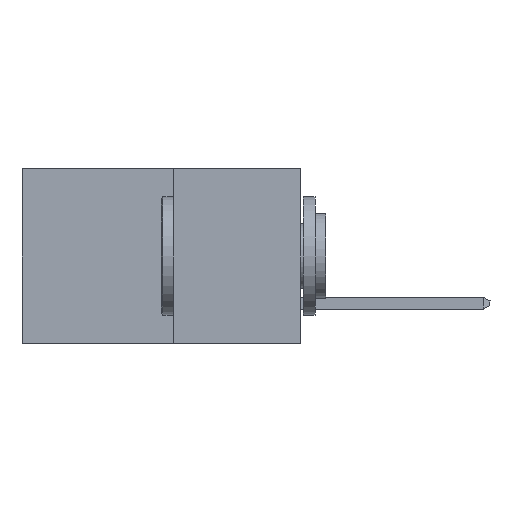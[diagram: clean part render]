
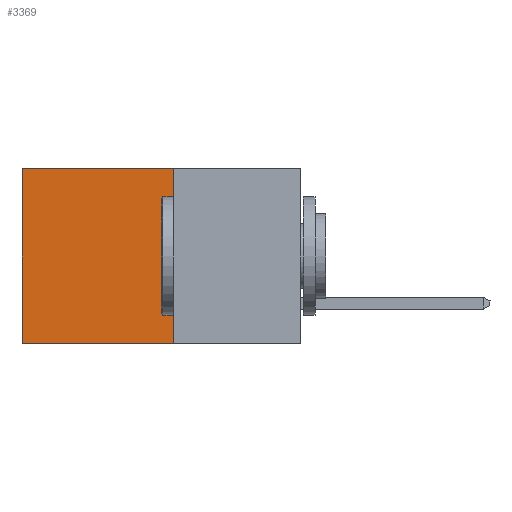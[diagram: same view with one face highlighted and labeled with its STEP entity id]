
A CAD part, left-side view. The second image highlights one B-rep face of the part: STEP entity #3369.
In plain terms, the highlighted planar face has unit normal (-1, 0, 0).
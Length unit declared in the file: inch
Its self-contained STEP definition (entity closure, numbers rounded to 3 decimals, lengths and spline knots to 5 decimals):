
#346 = VECTOR ( 'NONE', #9532, 39.37008 ) ;
#1127 = LINE ( 'NONE', #11704, #3586 ) ;
#1340 = VERTEX_POINT ( 'NONE', #4122 ) ;
#1895 = VERTEX_POINT ( 'NONE', #11166 ) ;
#2033 = ORIENTED_EDGE ( 'NONE', *, *, #8017, .T. ) ;
#2488 = EDGE_CURVE ( 'NONE', #5098, #1340, #13075, .T. ) ;
#2871 = CARTESIAN_POINT ( 'NONE',  ( 0.277, 0.27, -0.37 ) ) ;
#3369 = ADVANCED_FACE ( 'NONE', ( #10171 ), #11285, .F. ) ;
#3586 = VECTOR ( 'NONE', #9541, 39.37008 ) ;
#3850 = ORIENTED_EDGE ( 'NONE', *, *, #8998, .F. ) ;
#3867 = ORIENTED_EDGE ( 'NONE', *, *, #7310, .F. ) ;
#4122 = CARTESIAN_POINT ( 'NONE',  ( 0.277, 0.59, -0.37 ) ) ;
#4153 = EDGE_LOOP ( 'NONE', ( #10126, #3867, #3850, #2033 ) ) ;
#4335 = VECTOR ( 'NONE', #13903, 39.37008 ) ;
#5098 = VERTEX_POINT ( 'NONE', #14252 ) ;
#6669 = LINE ( 'NONE', #8452, #346 ) ;
#6967 = CARTESIAN_POINT ( 'NONE',  ( 0.277, 0.27, -0.37 ) ) ;
#7310 = EDGE_CURVE ( 'NONE', #8652, #1340, #7337, .T. ) ;
#7337 = LINE ( 'NONE', #2871, #4335 ) ;
#8017 = EDGE_CURVE ( 'NONE', #1895, #5098, #1127, .T. ) ;
#8452 = CARTESIAN_POINT ( 'NONE',  ( 0.277, 0.27, -0.37 ) ) ;
#8652 = VERTEX_POINT ( 'NONE', #6967 ) ;
#8998 = EDGE_CURVE ( 'NONE', #1895, #8652, #6669, .T. ) ;
#9532 = DIRECTION ( 'NONE',  ( 0., 0., -1. ) ) ;
#9541 = DIRECTION ( 'NONE',  ( 0., 1., 0. ) ) ;
#9862 = VECTOR ( 'NONE', #11952, 39.37008 ) ;
#9932 = AXIS2_PLACEMENT_3D ( 'NONE', #12037, #10806, #10727 ) ;
#10126 = ORIENTED_EDGE ( 'NONE', *, *, #2488, .T. ) ;
#10171 = FACE_OUTER_BOUND ( 'NONE', #4153, .T. ) ;
#10727 = DIRECTION ( 'NONE',  ( 0., 0., -1. ) ) ;
#10806 = DIRECTION ( 'NONE',  ( 1., 0., 0. ) ) ;
#11166 = CARTESIAN_POINT ( 'NONE',  ( 0.277, 0.27, 0. ) ) ;
#11285 = PLANE ( 'NONE',  #9932 ) ;
#11704 = CARTESIAN_POINT ( 'NONE',  ( 0.277, 0.27, 0. ) ) ;
#11767 = CARTESIAN_POINT ( 'NONE',  ( 0.277, 0.59, -0.37 ) ) ;
#11952 = DIRECTION ( 'NONE',  ( 0., 0., -1. ) ) ;
#12037 = CARTESIAN_POINT ( 'NONE',  ( 0.277, 0.27, -0.37 ) ) ;
#13075 = LINE ( 'NONE', #11767, #9862 ) ;
#13903 = DIRECTION ( 'NONE',  ( 0., 1., 0. ) ) ;
#14252 = CARTESIAN_POINT ( 'NONE',  ( 0.277, 0.59, 0. ) ) ;
